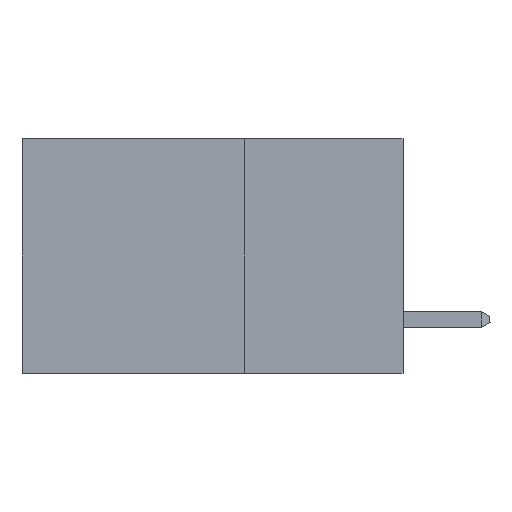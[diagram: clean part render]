
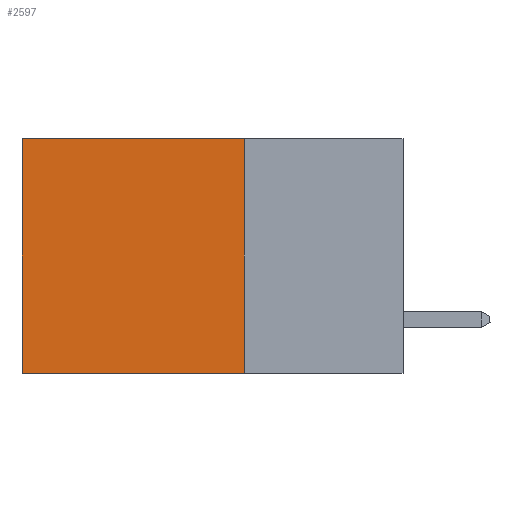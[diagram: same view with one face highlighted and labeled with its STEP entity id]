
A CAD part, left-side view. The second image highlights one B-rep face of the part: STEP entity #2597.
In plain terms, the highlighted planar face has unit normal (-1, 0, 0).
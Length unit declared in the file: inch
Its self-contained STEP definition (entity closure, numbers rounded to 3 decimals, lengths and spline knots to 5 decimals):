
#21 = ORIENTED_EDGE ( 'NONE', *, *, #7707, .F. ) ;
#90 = DIRECTION ( 'NONE',  ( 0., 0., -1. ) ) ;
#667 = VERTEX_POINT ( 'NONE', #9164 ) ;
#1271 = VECTOR ( 'NONE', #5631, 39.37008 ) ;
#1398 = CARTESIAN_POINT ( 'NONE',  ( 0.2875, 0.25, 0. ) ) ;
#1414 = CARTESIAN_POINT ( 'NONE',  ( 0.2875, 0.6, 0. ) ) ;
#1639 = LINE ( 'NONE', #1398, #6507 ) ;
#2597 = ADVANCED_FACE ( 'NONE', ( #4936 ), #4368, .F. ) ;
#3509 = LINE ( 'NONE', #8810, #13763 ) ;
#3831 = ORIENTED_EDGE ( 'NONE', *, *, #12755, .F. ) ;
#4176 = CARTESIAN_POINT ( 'NONE',  ( 0.2875, 0.6, 0. ) ) ;
#4214 = CARTESIAN_POINT ( 'NONE',  ( 0.2875, 0.25, 0. ) ) ;
#4368 = PLANE ( 'NONE',  #13510 ) ;
#4936 = FACE_OUTER_BOUND ( 'NONE', #12491, .T. ) ;
#5009 = VECTOR ( 'NONE', #10302, 39.37008 ) ;
#5075 = CARTESIAN_POINT ( 'NONE',  ( 0.2875, 0.25, 0. ) ) ;
#5631 = DIRECTION ( 'NONE',  ( 0., 0., -1. ) ) ;
#5948 = EDGE_CURVE ( 'NONE', #11857, #667, #11572, .T. ) ;
#6507 = VECTOR ( 'NONE', #90, 39.37008 ) ;
#7088 = EDGE_CURVE ( 'NONE', #9330, #11857, #7748, .T. ) ;
#7707 = EDGE_CURVE ( 'NONE', #9330, #8225, #1639, .T. ) ;
#7748 = LINE ( 'NONE', #5075, #5009 ) ;
#8225 = VERTEX_POINT ( 'NONE', #15655 ) ;
#8810 = CARTESIAN_POINT ( 'NONE',  ( 0.2875, 0.25, -0.37 ) ) ;
#8975 = DIRECTION ( 'NONE',  ( 0., 1., 0. ) ) ;
#9164 = CARTESIAN_POINT ( 'NONE',  ( 0.2875, 0.6, -0.37 ) ) ;
#9330 = VERTEX_POINT ( 'NONE', #4214 ) ;
#9418 = ORIENTED_EDGE ( 'NONE', *, *, #7088, .T. ) ;
#9812 = DIRECTION ( 'NONE',  ( 1., 0., 0. ) ) ;
#10302 = DIRECTION ( 'NONE',  ( 0., 1., 0. ) ) ;
#11162 = CARTESIAN_POINT ( 'NONE',  ( 0.2875, 0.25, 0. ) ) ;
#11572 = LINE ( 'NONE', #4176, #1271 ) ;
#11857 = VERTEX_POINT ( 'NONE', #1414 ) ;
#12491 = EDGE_LOOP ( 'NONE', ( #12929, #3831, #21, #9418 ) ) ;
#12755 = EDGE_CURVE ( 'NONE', #8225, #667, #3509, .T. ) ;
#12929 = ORIENTED_EDGE ( 'NONE', *, *, #5948, .T. ) ;
#13510 = AXIS2_PLACEMENT_3D ( 'NONE', #11162, #9812, #13796 ) ;
#13763 = VECTOR ( 'NONE', #8975, 39.37008 ) ;
#13796 = DIRECTION ( 'NONE',  ( 0., 0., -1. ) ) ;
#15655 = CARTESIAN_POINT ( 'NONE',  ( 0.2875, 0.25, -0.37 ) ) ;
